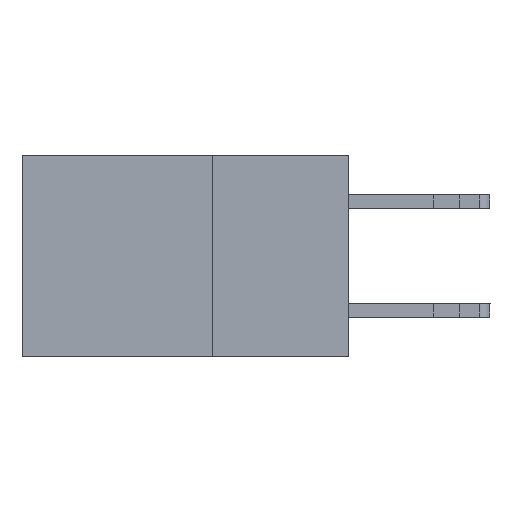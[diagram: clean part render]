
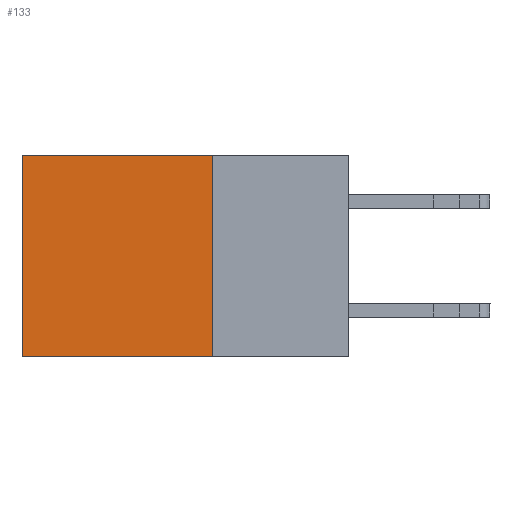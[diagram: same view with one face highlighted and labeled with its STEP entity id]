
A CAD part, left-side view. The second image highlights one B-rep face of the part: STEP entity #133.
In plain terms, the highlighted planar face has unit normal (-1, 0, 0).
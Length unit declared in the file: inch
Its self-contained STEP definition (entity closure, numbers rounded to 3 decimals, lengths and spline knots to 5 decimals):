
#107 = EDGE_CURVE ( 'NONE', #5614, #7566, #1382, .T. ) ;
#133 = ADVANCED_FACE ( 'NONE', ( #3480 ), #11421, .F. ) ;
#652 = EDGE_CURVE ( 'NONE', #4692, #7566, #5710, .T. ) ;
#1255 = DIRECTION ( 'NONE',  ( 0., 0., -1. ) ) ;
#1380 = CARTESIAN_POINT ( 'NONE',  ( 0.2615, 0.6, -0.37 ) ) ;
#1382 = LINE ( 'NONE', #1380, #3765 ) ;
#1396 = CARTESIAN_POINT ( 'NONE',  ( 0.2615, 0.6, -0.37 ) ) ;
#1592 = DIRECTION ( 'NONE',  ( 1., 0., 0. ) ) ;
#1724 = CARTESIAN_POINT ( 'NONE',  ( 0.2615, 0.25, 0. ) ) ;
#1773 = CARTESIAN_POINT ( 'NONE',  ( 0.2615, 0.25, -0.37 ) ) ;
#2403 = LINE ( 'NONE', #9358, #6907 ) ;
#2456 = DIRECTION ( 'NONE',  ( 0., 1., 0. ) ) ;
#3029 = EDGE_CURVE ( 'NONE', #4785, #5614, #2403, .T. ) ;
#3061 = VECTOR ( 'NONE', #5897, 39.37008 ) ;
#3480 = FACE_OUTER_BOUND ( 'NONE', #8505, .T. ) ;
#3765 = VECTOR ( 'NONE', #1255, 39.37008 ) ;
#4386 = DIRECTION ( 'NONE',  ( 0., 0., -1. ) ) ;
#4576 = EDGE_CURVE ( 'NONE', #4785, #4692, #5477, .T. ) ;
#4692 = VERTEX_POINT ( 'NONE', #10589 ) ;
#4785 = VERTEX_POINT ( 'NONE', #1724 ) ;
#5477 = LINE ( 'NONE', #10435, #3061 ) ;
#5614 = VERTEX_POINT ( 'NONE', #10039 ) ;
#5710 = LINE ( 'NONE', #1773, #10250 ) ;
#5897 = DIRECTION ( 'NONE',  ( 0., 0., -1. ) ) ;
#6907 = VECTOR ( 'NONE', #11137, 39.37008 ) ;
#7566 = VERTEX_POINT ( 'NONE', #1396 ) ;
#8421 = AXIS2_PLACEMENT_3D ( 'NONE', #8677, #1592, #4386 ) ;
#8505 = EDGE_LOOP ( 'NONE', ( #11180, #9062, #11457, #9345 ) ) ;
#8677 = CARTESIAN_POINT ( 'NONE',  ( 0.2615, 0.25, -0.37 ) ) ;
#9062 = ORIENTED_EDGE ( 'NONE', *, *, #652, .F. ) ;
#9345 = ORIENTED_EDGE ( 'NONE', *, *, #3029, .T. ) ;
#9358 = CARTESIAN_POINT ( 'NONE',  ( 0.2615, 0.25, 0. ) ) ;
#10039 = CARTESIAN_POINT ( 'NONE',  ( 0.2615, 0.6, 0. ) ) ;
#10250 = VECTOR ( 'NONE', #2456, 39.37008 ) ;
#10435 = CARTESIAN_POINT ( 'NONE',  ( 0.2615, 0.25, -0.37 ) ) ;
#10589 = CARTESIAN_POINT ( 'NONE',  ( 0.2615, 0.25, -0.37 ) ) ;
#11137 = DIRECTION ( 'NONE',  ( 0., 1., 0. ) ) ;
#11180 = ORIENTED_EDGE ( 'NONE', *, *, #107, .T. ) ;
#11421 = PLANE ( 'NONE',  #8421 ) ;
#11457 = ORIENTED_EDGE ( 'NONE', *, *, #4576, .F. ) ;
